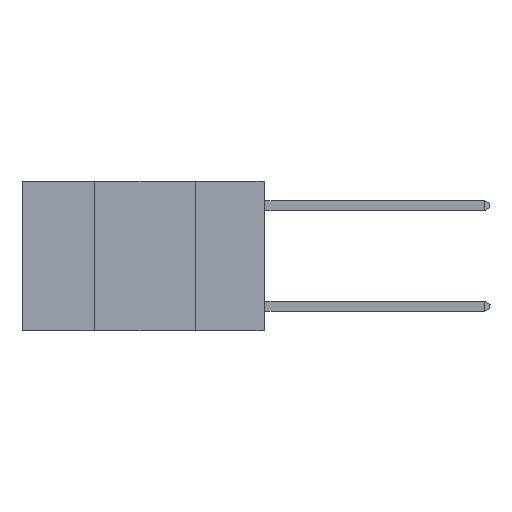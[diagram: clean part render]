
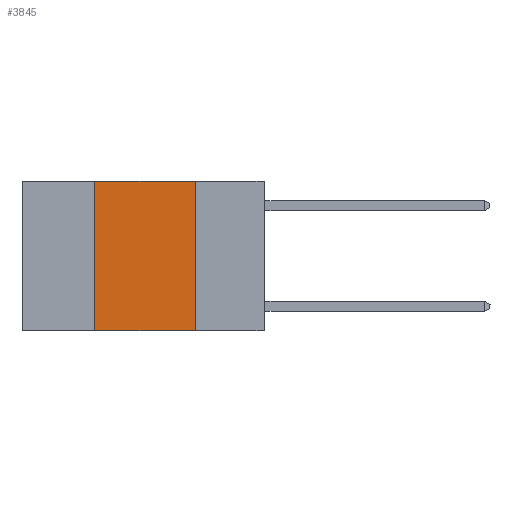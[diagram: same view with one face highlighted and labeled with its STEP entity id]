
A CAD part, left-side view. The second image highlights one B-rep face of the part: STEP entity #3845.
In plain terms, the highlighted planar face has unit normal (-1, 0, 0).
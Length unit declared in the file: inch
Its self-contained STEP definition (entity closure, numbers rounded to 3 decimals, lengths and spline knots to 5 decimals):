
#310 = VECTOR ( 'NONE', #18163, 39.37008 ) ;
#714 = CARTESIAN_POINT ( 'NONE',  ( 0., 0.6, 0. ) ) ;
#2681 = PLANE ( 'NONE',  #16614 ) ;
#2777 = VECTOR ( 'NONE', #12162, 39.37008 ) ;
#2970 = CARTESIAN_POINT ( 'NONE',  ( 0., 0.42, 0. ) ) ;
#3845 = ADVANCED_FACE ( 'NONE', ( #23407 ), #2681, .F. ) ;
#4557 = DIRECTION ( 'NONE',  ( 1., 0., 0. ) ) ;
#5037 = ORIENTED_EDGE ( 'NONE', *, *, #21814, .T. ) ;
#5456 = LINE ( 'NONE', #17975, #20798 ) ;
#6376 = CARTESIAN_POINT ( 'NONE',  ( 0., 0.17, 0. ) ) ;
#6440 = LINE ( 'NONE', #16321, #310 ) ;
#6646 = VERTEX_POINT ( 'NONE', #6376 ) ;
#8260 = LINE ( 'NONE', #2970, #2777 ) ;
#8890 = CARTESIAN_POINT ( 'NONE',  ( 0., 0.42, 0. ) ) ;
#11847 = CARTESIAN_POINT ( 'NONE',  ( 0., 0.17, -0.37 ) ) ;
#12162 = DIRECTION ( 'NONE',  ( 0., 0., 1. ) ) ;
#12349 = CARTESIAN_POINT ( 'NONE',  ( 0., 0.42, -0.37 ) ) ;
#12362 = EDGE_CURVE ( 'NONE', #6646, #15485, #19100, .T. ) ;
#12816 = ORIENTED_EDGE ( 'NONE', *, *, #12362, .F. ) ;
#12849 = DIRECTION ( 'NONE',  ( 0., 0., -1. ) ) ;
#13042 = EDGE_LOOP ( 'NONE', ( #12816, #20940, #16590, #5037 ) ) ;
#13376 = VERTEX_POINT ( 'NONE', #12349 ) ;
#15202 = VECTOR ( 'NONE', #12849, 39.37008 ) ;
#15485 = VERTEX_POINT ( 'NONE', #11847 ) ;
#15597 = EDGE_CURVE ( 'NONE', #13376, #16387, #8260, .T. ) ;
#16139 = DIRECTION ( 'NONE',  ( 0., -1., 0. ) ) ;
#16321 = CARTESIAN_POINT ( 'NONE',  ( 0., 0.6, 0. ) ) ;
#16387 = VERTEX_POINT ( 'NONE', #8890 ) ;
#16590 = ORIENTED_EDGE ( 'NONE', *, *, #15597, .F. ) ;
#16614 = AXIS2_PLACEMENT_3D ( 'NONE', #714, #4557, #17435 ) ;
#17435 = DIRECTION ( 'NONE',  ( 0., 0., -1. ) ) ;
#17975 = CARTESIAN_POINT ( 'NONE',  ( 0., 0.6, -0.37 ) ) ;
#18163 = DIRECTION ( 'NONE',  ( 0., -1., 0. ) ) ;
#18690 = EDGE_CURVE ( 'NONE', #16387, #6646, #6440, .T. ) ;
#19100 = LINE ( 'NONE', #23915, #15202 ) ;
#20798 = VECTOR ( 'NONE', #16139, 39.37008 ) ;
#20940 = ORIENTED_EDGE ( 'NONE', *, *, #18690, .F. ) ;
#21814 = EDGE_CURVE ( 'NONE', #13376, #15485, #5456, .T. ) ;
#23407 = FACE_OUTER_BOUND ( 'NONE', #13042, .T. ) ;
#23915 = CARTESIAN_POINT ( 'NONE',  ( 0., 0.17, 0. ) ) ;
